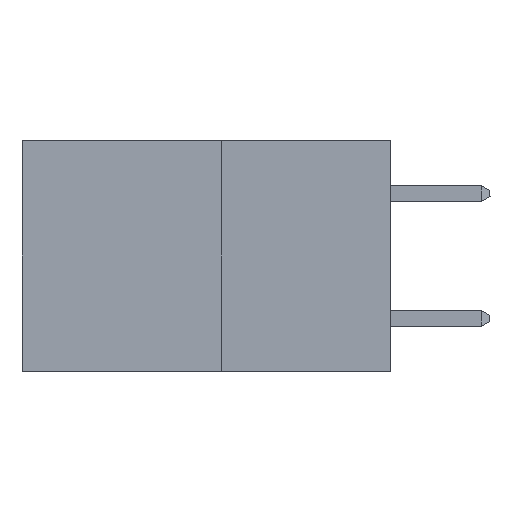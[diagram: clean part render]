
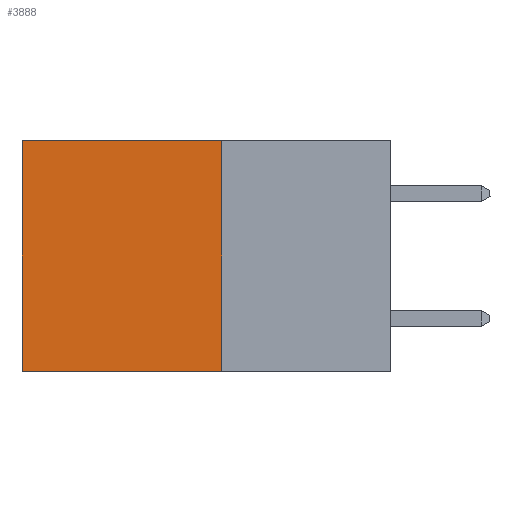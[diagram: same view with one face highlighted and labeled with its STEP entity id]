
A CAD part, left-side view. The second image highlights one B-rep face of the part: STEP entity #3888.
In plain terms, the highlighted planar face has unit normal (-1, 0, 0).
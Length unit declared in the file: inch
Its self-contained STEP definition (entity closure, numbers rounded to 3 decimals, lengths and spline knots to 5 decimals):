
#478 = DIRECTION ( 'NONE',  ( 0., 0., -1. ) ) ;
#574 = EDGE_LOOP ( 'NONE', ( #5912, #11040, #12574, #14518 ) ) ;
#949 = CARTESIAN_POINT ( 'NONE',  ( 0.277, 0.27, 0. ) ) ;
#1334 = DIRECTION ( 'NONE',  ( 1., 0., 0. ) ) ;
#2234 = CARTESIAN_POINT ( 'NONE',  ( 0.277, 0.27, -0.37 ) ) ;
#3487 = EDGE_CURVE ( 'NONE', #16210, #11100, #3999, .T. ) ;
#3888 = ADVANCED_FACE ( 'NONE', ( #15735 ), #7038, .F. ) ;
#3999 = LINE ( 'NONE', #11224, #11273 ) ;
#5099 = CARTESIAN_POINT ( 'NONE',  ( 0.277, 0.59, -0.37 ) ) ;
#5582 = CARTESIAN_POINT ( 'NONE',  ( 0.277, 0.27, -0.37 ) ) ;
#5912 = ORIENTED_EDGE ( 'NONE', *, *, #10822, .T. ) ;
#6250 = DIRECTION ( 'NONE',  ( 0., 1., 0. ) ) ;
#6365 = CARTESIAN_POINT ( 'NONE',  ( 0.277, 0.27, 0. ) ) ;
#6494 = AXIS2_PLACEMENT_3D ( 'NONE', #5582, #1334, #17243 ) ;
#7038 = PLANE ( 'NONE',  #6494 ) ;
#7435 = VECTOR ( 'NONE', #14777, 39.37008 ) ;
#8108 = LINE ( 'NONE', #6365, #14972 ) ;
#8290 = VERTEX_POINT ( 'NONE', #15535 ) ;
#8416 = EDGE_CURVE ( 'NONE', #11100, #10191, #11070, .T. ) ;
#10191 = VERTEX_POINT ( 'NONE', #5099 ) ;
#10822 = EDGE_CURVE ( 'NONE', #8290, #10191, #14678, .T. ) ;
#11040 = ORIENTED_EDGE ( 'NONE', *, *, #8416, .F. ) ;
#11070 = LINE ( 'NONE', #2234, #7435 ) ;
#11100 = VERTEX_POINT ( 'NONE', #11333 ) ;
#11224 = CARTESIAN_POINT ( 'NONE',  ( 0.277, 0.27, -0.37 ) ) ;
#11273 = VECTOR ( 'NONE', #478, 39.37008 ) ;
#11333 = CARTESIAN_POINT ( 'NONE',  ( 0.277, 0.27, -0.37 ) ) ;
#11450 = VECTOR ( 'NONE', #15891, 39.37008 ) ;
#12574 = ORIENTED_EDGE ( 'NONE', *, *, #3487, .F. ) ;
#14029 = EDGE_CURVE ( 'NONE', #16210, #8290, #8108, .T. ) ;
#14518 = ORIENTED_EDGE ( 'NONE', *, *, #14029, .T. ) ;
#14678 = LINE ( 'NONE', #15639, #11450 ) ;
#14777 = DIRECTION ( 'NONE',  ( 0., 1., 0. ) ) ;
#14972 = VECTOR ( 'NONE', #6250, 39.37008 ) ;
#15535 = CARTESIAN_POINT ( 'NONE',  ( 0.277, 0.59, 0. ) ) ;
#15639 = CARTESIAN_POINT ( 'NONE',  ( 0.277, 0.59, -0.37 ) ) ;
#15735 = FACE_OUTER_BOUND ( 'NONE', #574, .T. ) ;
#15891 = DIRECTION ( 'NONE',  ( 0., 0., -1. ) ) ;
#16210 = VERTEX_POINT ( 'NONE', #949 ) ;
#17243 = DIRECTION ( 'NONE',  ( 0., 0., -1. ) ) ;
